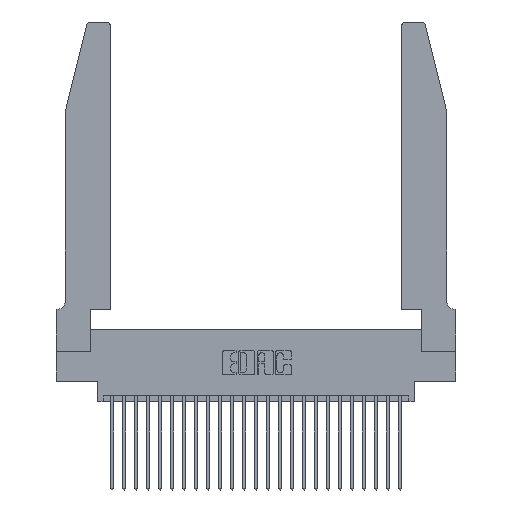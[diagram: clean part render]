
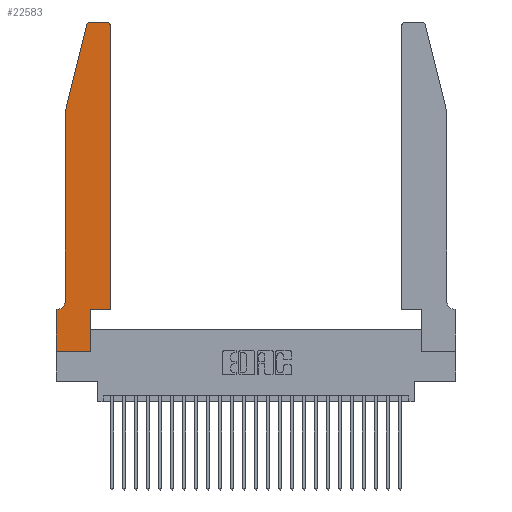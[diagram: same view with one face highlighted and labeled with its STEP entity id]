
A CAD part, top view. The second image highlights one B-rep face of the part: STEP entity #22583.
In plain terms, the highlighted planar face has unit normal (0, 0, 1).
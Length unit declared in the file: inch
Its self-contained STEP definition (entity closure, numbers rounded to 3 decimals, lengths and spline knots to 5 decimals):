
#1 = LINE ( 'NONE', #25255, #4976 ) ;
#206 = VERTEX_POINT ( 'NONE', #8991 ) ;
#470 = CARTESIAN_POINT ( 'NONE',  ( 0.284, 2.72, 0.37 ) ) ;
#832 = LINE ( 'NONE', #7071, #21656 ) ;
#991 = DIRECTION ( 'NONE',  ( -1., 0., 0. ) ) ;
#1166 = DIRECTION ( 'NONE',  ( -1., 0., 0. ) ) ;
#1332 = EDGE_CURVE ( 'NONE', #9497, #9685, #10707, .T. ) ;
#1635 = CARTESIAN_POINT ( 'NONE',  ( 0.0755, 2., 0.37 ) ) ;
#1947 = DIRECTION ( 'NONE',  ( 1., 0., 0. ) ) ;
#2043 = EDGE_CURVE ( 'NONE', #4126, #25773, #1, .T. ) ;
#2232 = CARTESIAN_POINT ( 'NONE',  ( 0.4205, 2.72, 0.37 ) ) ;
#2576 = DIRECTION ( 'NONE',  ( 1., 0., 0. ) ) ;
#3401 = CARTESIAN_POINT ( 'NONE',  ( 0.4505, 0.35, 0.37 ) ) ;
#3918 = VERTEX_POINT ( 'NONE', #10070 ) ;
#4126 = VERTEX_POINT ( 'NONE', #6501 ) ;
#4157 = EDGE_LOOP ( 'NONE', ( #4931, #24364, #25615, #25351, #18603, #17306, #25644, #7924, #12155, #8976, #26724, #25211 ) ) ;
#4336 = VERTEX_POINT ( 'NONE', #25678 ) ;
#4371 = DIRECTION ( 'NONE',  ( 1., 0., 0. ) ) ;
#4931 = ORIENTED_EDGE ( 'NONE', *, *, #19094, .T. ) ;
#4976 = VECTOR ( 'NONE', #10347, 39.37008 ) ;
#5536 = VERTEX_POINT ( 'NONE', #23203 ) ;
#5819 = CIRCLE ( 'NONE', #17356, 0.03 ) ;
#6192 = CARTESIAN_POINT ( 'NONE',  ( 0.0755, 2., 0.37 ) ) ;
#6255 = CARTESIAN_POINT ( 'NONE',  ( 0., 0., 0.37 ) ) ;
#6306 = VERTEX_POINT ( 'NONE', #15413 ) ;
#6501 = CARTESIAN_POINT ( 'NONE',  ( 0.25487, 2.72718, 0.37 ) ) ;
#6535 = DIRECTION ( 'NONE',  ( 0., 1., 0. ) ) ;
#7071 = CARTESIAN_POINT ( 'NONE',  ( 0.2865, 0.35, 0.37 ) ) ;
#7176 = VECTOR ( 'NONE', #6535, 39.37008 ) ;
#7787 = CARTESIAN_POINT ( 'NONE',  ( 0.4505, 0.35, 0.37 ) ) ;
#7924 = ORIENTED_EDGE ( 'NONE', *, *, #1332, .T. ) ;
#8529 = EDGE_CURVE ( 'NONE', #3918, #206, #22016, .T. ) ;
#8976 = ORIENTED_EDGE ( 'NONE', *, *, #12435, .T. ) ;
#8991 = CARTESIAN_POINT ( 'NONE',  ( 0.4205, 2.75, 0.37 ) ) ;
#9378 = VECTOR ( 'NONE', #13529, 39.37008 ) ;
#9497 = VERTEX_POINT ( 'NONE', #6255 ) ;
#9685 = VERTEX_POINT ( 'NONE', #10975 ) ;
#9916 = AXIS2_PLACEMENT_3D ( 'NONE', #2232, #16802, #4371 ) ;
#10070 = CARTESIAN_POINT ( 'NONE',  ( 0.4505, 2.72, 0.37 ) ) ;
#10347 = DIRECTION ( 'NONE',  ( -0.239, -0.971, 0. ) ) ;
#10593 = LINE ( 'NONE', #10802, #16723 ) ;
#10707 = LINE ( 'NONE', #23193, #16195 ) ;
#10802 = CARTESIAN_POINT ( 'NONE',  ( 0., 0., 0.37 ) ) ;
#10858 = VECTOR ( 'NONE', #18292, 39.37008 ) ;
#10975 = CARTESIAN_POINT ( 'NONE',  ( 0.2865, 0., 0.37 ) ) ;
#10978 = VERTEX_POINT ( 'NONE', #13673 ) ;
#11843 = EDGE_CURVE ( 'NONE', #25773, #4336, #21830, .T. ) ;
#12155 = ORIENTED_EDGE ( 'NONE', *, *, #21453, .T. ) ;
#12397 = PLANE ( 'NONE',  #25637 ) ;
#12435 = EDGE_CURVE ( 'NONE', #10978, #21708, #24685, .T. ) ;
#12594 = AXIS2_PLACEMENT_3D ( 'NONE', #25834, #13561, #991 ) ;
#13357 = DIRECTION ( 'NONE',  ( 0., 1., 0. ) ) ;
#13529 = DIRECTION ( 'NONE',  ( -1., 0., 0. ) ) ;
#13561 = DIRECTION ( 'NONE',  ( 0., 0., -1. ) ) ;
#13673 = CARTESIAN_POINT ( 'NONE',  ( 0.2865, 0.35, 0.37 ) ) ;
#14409 = VECTOR ( 'NONE', #17937, 39.37008 ) ;
#14469 = DIRECTION ( 'NONE',  ( 0., 0., 1. ) ) ;
#15081 = DIRECTION ( 'NONE',  ( 0., 0., 1. ) ) ;
#15413 = CARTESIAN_POINT ( 'NONE',  ( 0.284, 2.75, 0.37 ) ) ;
#15429 = EDGE_CURVE ( 'NONE', #22265, #9497, #10593, .T. ) ;
#15600 = CARTESIAN_POINT ( 'NONE',  ( 0.0755, 0.35, 0.37 ) ) ;
#16195 = VECTOR ( 'NONE', #23138, 39.37008 ) ;
#16531 = VECTOR ( 'NONE', #1166, 39.37008 ) ;
#16723 = VECTOR ( 'NONE', #16943, 39.37008 ) ;
#16802 = DIRECTION ( 'NONE',  ( 0., 0., 1. ) ) ;
#16943 = DIRECTION ( 'NONE',  ( 0., -1., 0. ) ) ;
#17306 = ORIENTED_EDGE ( 'NONE', *, *, #21526, .T. ) ;
#17356 = AXIS2_PLACEMENT_3D ( 'NONE', #470, #15081, #2576 ) ;
#17604 = CARTESIAN_POINT ( 'NONE',  ( 0., 0.35, 0.37 ) ) ;
#17714 = FACE_OUTER_BOUND ( 'NONE', #4157, .T. ) ;
#17937 = DIRECTION ( 'NONE',  ( 1., 0., 0. ) ) ;
#18165 = LINE ( 'NONE', #23079, #7176 ) ;
#18292 = DIRECTION ( 'NONE',  ( 0., -1., 0. ) ) ;
#18603 = ORIENTED_EDGE ( 'NONE', *, *, #23611, .T. ) ;
#18806 = EDGE_CURVE ( 'NONE', #21708, #3918, #18165, .T. ) ;
#19094 = EDGE_CURVE ( 'NONE', #206, #6306, #22025, .T. ) ;
#19794 = EDGE_CURVE ( 'NONE', #6306, #4126, #5819, .T. ) ;
#20573 = CARTESIAN_POINT ( 'NONE',  ( 0., 0.35, 0.37 ) ) ;
#21206 = CIRCLE ( 'NONE', #12594, 0.07 ) ;
#21453 = EDGE_CURVE ( 'NONE', #9685, #10978, #832, .T. ) ;
#21526 = EDGE_CURVE ( 'NONE', #5536, #22265, #25799, .T. ) ;
#21656 = VECTOR ( 'NONE', #13357, 39.37008 ) ;
#21708 = VERTEX_POINT ( 'NONE', #7787 ) ;
#21830 = LINE ( 'NONE', #1635, #10858 ) ;
#21895 = CARTESIAN_POINT ( 'NONE',  ( 0.2605, 2.75, 0.37 ) ) ;
#22016 = CIRCLE ( 'NONE', #9916, 0.03 ) ;
#22025 = LINE ( 'NONE', #21895, #16531 ) ;
#22265 = VERTEX_POINT ( 'NONE', #17604 ) ;
#22583 = ADVANCED_FACE ( 'NONE', ( #17714 ), #12397, .T. ) ;
#23079 = CARTESIAN_POINT ( 'NONE',  ( 0.4505, 0.35, 0.37 ) ) ;
#23138 = DIRECTION ( 'NONE',  ( 1., 0., 0. ) ) ;
#23193 = CARTESIAN_POINT ( 'NONE',  ( 0., 0., 0.37 ) ) ;
#23203 = CARTESIAN_POINT ( 'NONE',  ( 0.0055, 0.35, 0.37 ) ) ;
#23611 = EDGE_CURVE ( 'NONE', #4336, #5536, #21206, .T. ) ;
#24364 = ORIENTED_EDGE ( 'NONE', *, *, #19794, .T. ) ;
#24685 = LINE ( 'NONE', #3401, #14409 ) ;
#25211 = ORIENTED_EDGE ( 'NONE', *, *, #8529, .T. ) ;
#25255 = CARTESIAN_POINT ( 'NONE',  ( 0.0755, 2., 0.37 ) ) ;
#25351 = ORIENTED_EDGE ( 'NONE', *, *, #11843, .T. ) ;
#25615 = ORIENTED_EDGE ( 'NONE', *, *, #2043, .T. ) ;
#25637 = AXIS2_PLACEMENT_3D ( 'NONE', #20573, #14469, #1947 ) ;
#25644 = ORIENTED_EDGE ( 'NONE', *, *, #15429, .T. ) ;
#25678 = CARTESIAN_POINT ( 'NONE',  ( 0.0755, 0.42, 0.37 ) ) ;
#25773 = VERTEX_POINT ( 'NONE', #6192 ) ;
#25799 = LINE ( 'NONE', #15600, #9378 ) ;
#25834 = CARTESIAN_POINT ( 'NONE',  ( 0.0055, 0.42, 0.37 ) ) ;
#26724 = ORIENTED_EDGE ( 'NONE', *, *, #18806, .T. ) ;
